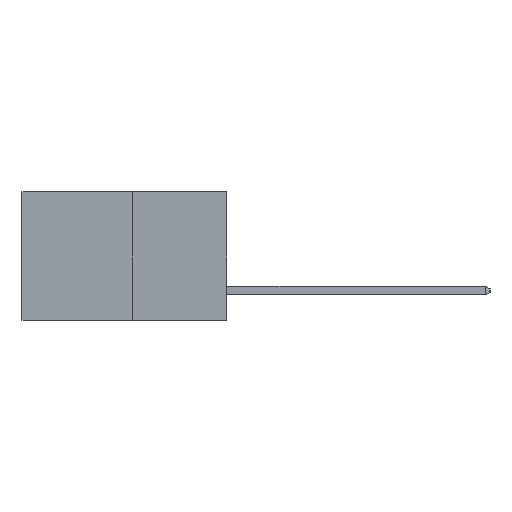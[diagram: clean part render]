
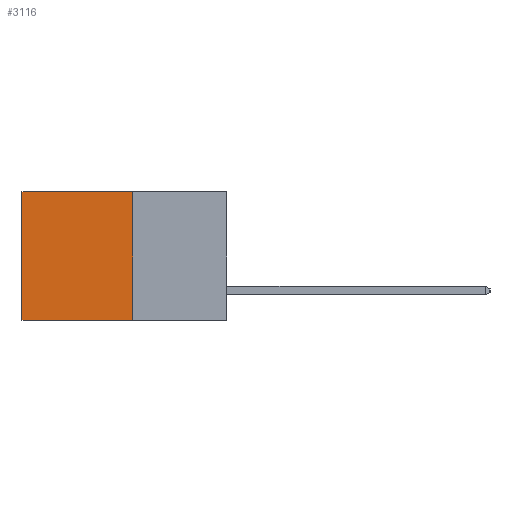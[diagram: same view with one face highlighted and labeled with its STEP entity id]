
A CAD part, left-side view. The second image highlights one B-rep face of the part: STEP entity #3116.
In plain terms, the highlighted planar face has unit normal (-1, 0, 0).
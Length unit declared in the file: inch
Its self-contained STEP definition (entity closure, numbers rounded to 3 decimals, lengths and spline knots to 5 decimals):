
#168 = VERTEX_POINT ( 'NONE', #9390 ) ;
#616 = CARTESIAN_POINT ( 'NONE',  ( 0.277, 0.59, 0. ) ) ;
#617 = ORIENTED_EDGE ( 'NONE', *, *, #2730, .T. ) ;
#680 = VECTOR ( 'NONE', #4766, 39.37008 ) ;
#900 = DIRECTION ( 'NONE',  ( 0., 0., -1. ) ) ;
#970 = ORIENTED_EDGE ( 'NONE', *, *, #3404, .F. ) ;
#1050 = VECTOR ( 'NONE', #6485, 39.37008 ) ;
#1510 = VERTEX_POINT ( 'NONE', #2484 ) ;
#1955 = EDGE_CURVE ( 'NONE', #1510, #7369, #2956, .T. ) ;
#2223 = LINE ( 'NONE', #7321, #680 ) ;
#2446 = VERTEX_POINT ( 'NONE', #616 ) ;
#2484 = CARTESIAN_POINT ( 'NONE',  ( 0.277, 0.27, 0. ) ) ;
#2561 = ORIENTED_EDGE ( 'NONE', *, *, #6671, .T. ) ;
#2730 = EDGE_CURVE ( 'NONE', #1510, #2446, #4332, .T. ) ;
#2956 = LINE ( 'NONE', #5147, #4697 ) ;
#3116 = ADVANCED_FACE ( 'NONE', ( #3516 ), #3564, .F. ) ;
#3165 = LINE ( 'NONE', #8569, #8648 ) ;
#3404 = EDGE_CURVE ( 'NONE', #7369, #168, #3165, .T. ) ;
#3516 = FACE_OUTER_BOUND ( 'NONE', #7767, .T. ) ;
#3564 = PLANE ( 'NONE',  #9200 ) ;
#3635 = CARTESIAN_POINT ( 'NONE',  ( 0.277, 0.27, -0.37 ) ) ;
#3664 = DIRECTION ( 'NONE',  ( 1., 0., 0. ) ) ;
#3715 = CARTESIAN_POINT ( 'NONE',  ( 0.277, 0.27, -0.37 ) ) ;
#4332 = LINE ( 'NONE', #6493, #1050 ) ;
#4697 = VECTOR ( 'NONE', #8007, 39.37008 ) ;
#4766 = DIRECTION ( 'NONE',  ( 0., 0., -1. ) ) ;
#5147 = CARTESIAN_POINT ( 'NONE',  ( 0.277, 0.27, -0.37 ) ) ;
#6485 = DIRECTION ( 'NONE',  ( 0., 1., 0. ) ) ;
#6493 = CARTESIAN_POINT ( 'NONE',  ( 0.277, 0.27, 0. ) ) ;
#6671 = EDGE_CURVE ( 'NONE', #2446, #168, #2223, .T. ) ;
#7321 = CARTESIAN_POINT ( 'NONE',  ( 0.277, 0.59, -0.37 ) ) ;
#7369 = VERTEX_POINT ( 'NONE', #3635 ) ;
#7767 = EDGE_LOOP ( 'NONE', ( #2561, #970, #9407, #617 ) ) ;
#8007 = DIRECTION ( 'NONE',  ( 0., 0., -1. ) ) ;
#8064 = DIRECTION ( 'NONE',  ( 0., 1., 0. ) ) ;
#8569 = CARTESIAN_POINT ( 'NONE',  ( 0.277, 0.27, -0.37 ) ) ;
#8648 = VECTOR ( 'NONE', #8064, 39.37008 ) ;
#9200 = AXIS2_PLACEMENT_3D ( 'NONE', #3715, #3664, #900 ) ;
#9390 = CARTESIAN_POINT ( 'NONE',  ( 0.277, 0.59, -0.37 ) ) ;
#9407 = ORIENTED_EDGE ( 'NONE', *, *, #1955, .F. ) ;
